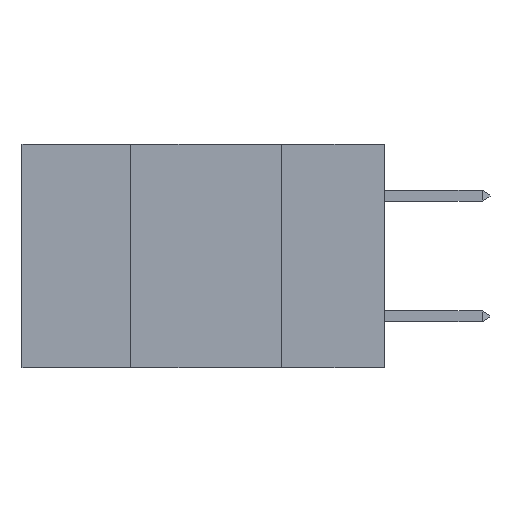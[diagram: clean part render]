
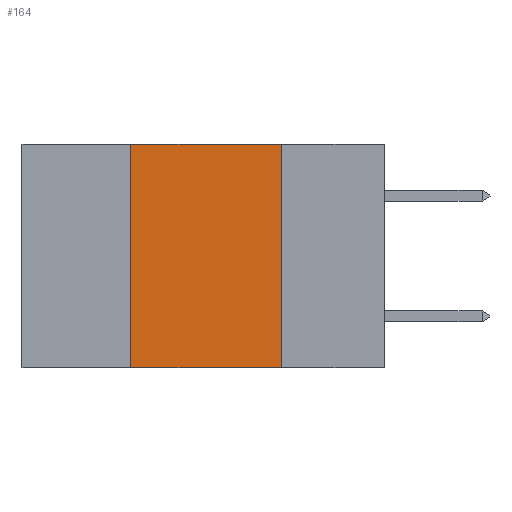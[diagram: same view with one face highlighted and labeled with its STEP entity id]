
A CAD part, left-side view. The second image highlights one B-rep face of the part: STEP entity #164.
In plain terms, the highlighted planar face has unit normal (-1, 0, 0).
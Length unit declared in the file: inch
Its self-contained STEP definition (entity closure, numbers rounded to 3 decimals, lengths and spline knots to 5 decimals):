
#161 = EDGE_CURVE ( 'NONE', #9602, #5776, #1849, .T. ) ;
#164 = ADVANCED_FACE ( 'NONE', ( #1770 ), #8947, .F. ) ;
#570 = LINE ( 'NONE', #9073, #12107 ) ;
#606 = DIRECTION ( 'NONE',  ( 1., 0., 0. ) ) ;
#1095 = ORIENTED_EDGE ( 'NONE', *, *, #5123, .F. ) ;
#1210 = EDGE_CURVE ( 'NONE', #4415, #3834, #570, .T. ) ;
#1365 = ORIENTED_EDGE ( 'NONE', *, *, #15234, .F. ) ;
#1770 = FACE_OUTER_BOUND ( 'NONE', #2412, .T. ) ;
#1849 = LINE ( 'NONE', #14982, #10954 ) ;
#2009 = LINE ( 'NONE', #3111, #6080 ) ;
#2412 = EDGE_LOOP ( 'NONE', ( #1365, #3511, #1095, #3922 ) ) ;
#2417 = CARTESIAN_POINT ( 'NONE',  ( 0., 0.42, 0. ) ) ;
#3111 = CARTESIAN_POINT ( 'NONE',  ( 0., 0.42, 0. ) ) ;
#3511 = ORIENTED_EDGE ( 'NONE', *, *, #1210, .F. ) ;
#3834 = VERTEX_POINT ( 'NONE', #7902 ) ;
#3922 = ORIENTED_EDGE ( 'NONE', *, *, #161, .T. ) ;
#4415 = VERTEX_POINT ( 'NONE', #2417 ) ;
#5123 = EDGE_CURVE ( 'NONE', #9602, #4415, #2009, .T. ) ;
#5349 = CARTESIAN_POINT ( 'NONE',  ( 0., 0.17, 0. ) ) ;
#5776 = VERTEX_POINT ( 'NONE', #13041 ) ;
#6080 = VECTOR ( 'NONE', #10352, 39.37008 ) ;
#7239 = CARTESIAN_POINT ( 'NONE',  ( 0., 0.42, -0.37 ) ) ;
#7902 = CARTESIAN_POINT ( 'NONE',  ( 0., 0.17, 0. ) ) ;
#8092 = DIRECTION ( 'NONE',  ( 0., -1., 0. ) ) ;
#8947 = PLANE ( 'NONE',  #13208 ) ;
#9072 = DIRECTION ( 'NONE',  ( 0., 0., -1. ) ) ;
#9073 = CARTESIAN_POINT ( 'NONE',  ( 0., 0.6, 0. ) ) ;
#9602 = VERTEX_POINT ( 'NONE', #7239 ) ;
#10116 = DIRECTION ( 'NONE',  ( 0., 0., -1. ) ) ;
#10198 = DIRECTION ( 'NONE',  ( 0., -1., 0. ) ) ;
#10352 = DIRECTION ( 'NONE',  ( 0., 0., 1. ) ) ;
#10452 = VECTOR ( 'NONE', #9072, 39.37008 ) ;
#10954 = VECTOR ( 'NONE', #10198, 39.37008 ) ;
#11302 = CARTESIAN_POINT ( 'NONE',  ( 0., 0.6, 0. ) ) ;
#12107 = VECTOR ( 'NONE', #8092, 39.37008 ) ;
#13041 = CARTESIAN_POINT ( 'NONE',  ( 0., 0.17, -0.37 ) ) ;
#13208 = AXIS2_PLACEMENT_3D ( 'NONE', #11302, #606, #10116 ) ;
#14982 = CARTESIAN_POINT ( 'NONE',  ( 0., 0.6, -0.37 ) ) ;
#15097 = LINE ( 'NONE', #5349, #10452 ) ;
#15234 = EDGE_CURVE ( 'NONE', #3834, #5776, #15097, .T. ) ;
